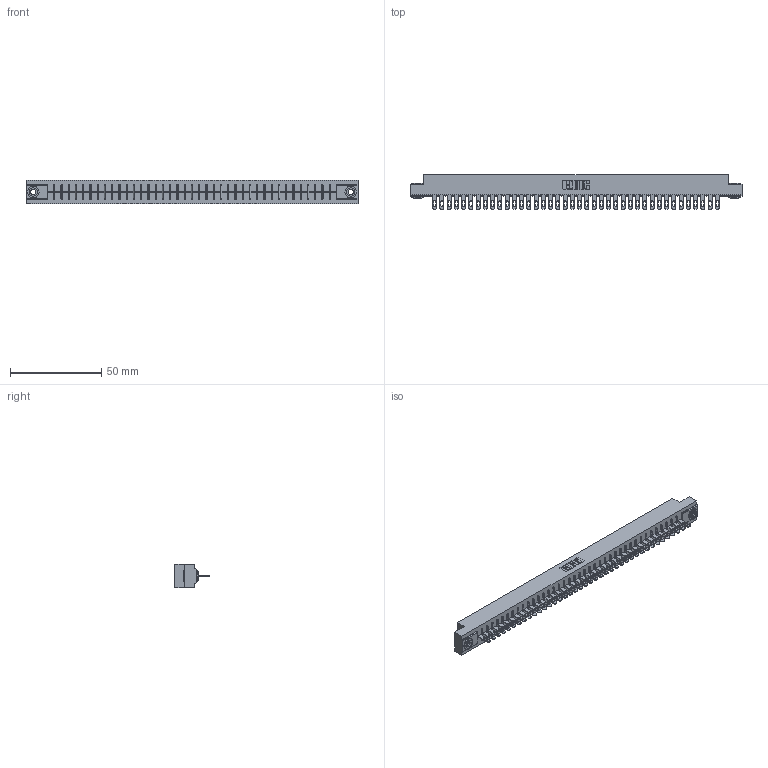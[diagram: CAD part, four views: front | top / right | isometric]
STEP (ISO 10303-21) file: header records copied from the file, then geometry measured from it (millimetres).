
FILE_DESCRIPTION (( 'STEP AP203' ), '1' );
FILE_NAME ('316-040-400-103.STEP', '2020-09-23T06:31:46', ( '' ), ( '' ), 'SwSTEP 2.0', 'SolidWorks 2020', '' );
FILE_SCHEMA (( 'CONFIG_CONTROL_DESIGN' ));
Length unit declared in the file: inch
Products named in the file (4): 345-250-002_345-250-002-102; 306 Part_.156 Dia; 316-040-400-103; 306-290-001_100
Assembly tree (43 placements, depth 2):
  316-040-400-103
    306 Part_.156 Dia
    306-290-001_100  x40
    345-250-002_345-250-002-102  x2
Bounding box: 181.51 x 18.87 x 12.7 mm (x, y, z)
Volume: 20192.3 mm3; surface area: 21650.7 mm2
Topology: 43 solids, 43 shells, 3208 faces, 9028 edges, 5800 vertices
Faces by surface type: plane 2092, cylinder 948, sphere 160, cone 8
Entity records: 38790 total; most frequent: CARTESIAN_POINT 6492, ORIENTED_EDGE 6428, DIRECTION 6416, EDGE_CURVE 3214, LINE 2504, VECTOR 2504, VERTEX_POINT 2032, AXIS2_PLACEMENT_3D 1956
